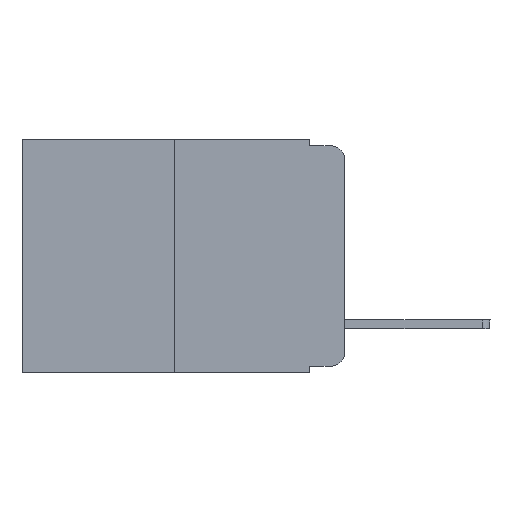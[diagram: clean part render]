
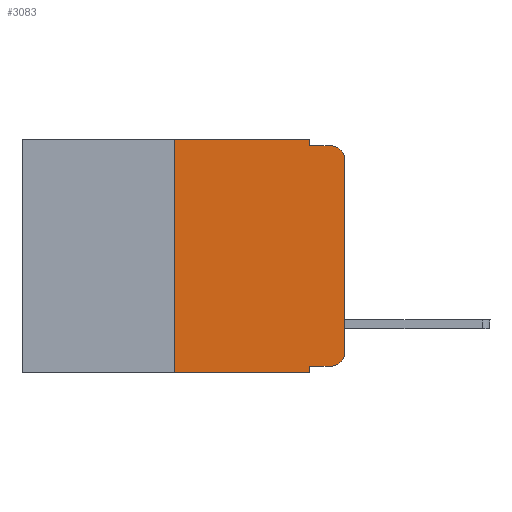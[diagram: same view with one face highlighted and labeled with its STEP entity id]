
A CAD part, left-side view. The second image highlights one B-rep face of the part: STEP entity #3083.
In plain terms, the highlighted planar face has unit normal (-1, 0, 0).
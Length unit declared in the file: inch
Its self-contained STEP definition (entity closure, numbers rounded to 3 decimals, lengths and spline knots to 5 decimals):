
#140 = DIRECTION ( 'NONE',  ( 0., -1., 0. ) ) ;
#408 = VERTEX_POINT ( 'NONE', #910 ) ;
#553 = ORIENTED_EDGE ( 'NONE', *, *, #4506, .T. ) ;
#562 = LINE ( 'NONE', #4885, #9786 ) ;
#564 = DIRECTION ( 'NONE',  ( 1., 0., 0. ) ) ;
#711 = EDGE_LOOP ( 'NONE', ( #5844, #2685, #13274, #2821, #1053, #6783, #12156, #6598, #553, #3997 ) ) ;
#843 = VERTEX_POINT ( 'NONE', #11855 ) ;
#910 = CARTESIAN_POINT ( 'NONE',  ( 0., 0.051, -0.01 ) ) ;
#1053 = ORIENTED_EDGE ( 'NONE', *, *, #3729, .F. ) ;
#1179 = VECTOR ( 'NONE', #4128, 39.37008 ) ;
#1207 = DIRECTION ( 'NONE',  ( 0., 0., -1. ) ) ;
#1239 = CARTESIAN_POINT ( 'NONE',  ( 0., 0.051, -0.333 ) ) ;
#1391 = CARTESIAN_POINT ( 'NONE',  ( 0., 0.25, 0. ) ) ;
#1409 = DIRECTION ( 'NONE',  ( 0., -1., 0. ) ) ;
#1519 = EDGE_CURVE ( 'NONE', #1644, #10442, #2931, .T. ) ;
#1644 = VERTEX_POINT ( 'NONE', #6235 ) ;
#1645 = DIRECTION ( 'NONE',  ( 0., -1., 0. ) ) ;
#1704 = VERTEX_POINT ( 'NONE', #1391 ) ;
#1884 = EDGE_CURVE ( 'NONE', #9315, #13483, #562, .T. ) ;
#2300 = LINE ( 'NONE', #12672, #10249 ) ;
#2417 = LINE ( 'NONE', #4503, #10703 ) ;
#2685 = ORIENTED_EDGE ( 'NONE', *, *, #12459, .T. ) ;
#2821 = ORIENTED_EDGE ( 'NONE', *, *, #6728, .F. ) ;
#2931 = CIRCLE ( 'NONE', #3819, 0.02 ) ;
#3071 = LINE ( 'NONE', #3214, #1179 ) ;
#3083 = ADVANCED_FACE ( 'NONE', ( #5799 ), #9998, .F. ) ;
#3214 = CARTESIAN_POINT ( 'NONE',  ( 0., 0.051, -0.01 ) ) ;
#3233 = CARTESIAN_POINT ( 'NONE',  ( 0., 0., -0.313 ) ) ;
#3527 = CARTESIAN_POINT ( 'NONE',  ( 0., 0.473, 0. ) ) ;
#3534 = LINE ( 'NONE', #6016, #8537 ) ;
#3564 = CARTESIAN_POINT ( 'NONE',  ( 0., 0.25, -0.343 ) ) ;
#3729 = EDGE_CURVE ( 'NONE', #1704, #4310, #6667, .T. ) ;
#3819 = AXIS2_PLACEMENT_3D ( 'NONE', #13474, #7956, #11334 ) ;
#3989 = EDGE_CURVE ( 'NONE', #8531, #13483, #2417, .T. ) ;
#3997 = ORIENTED_EDGE ( 'NONE', *, *, #1519, .T. ) ;
#4117 = AXIS2_PLACEMENT_3D ( 'NONE', #3527, #564, #7755 ) ;
#4128 = DIRECTION ( 'NONE',  ( 0., -1., 0. ) ) ;
#4310 = VERTEX_POINT ( 'NONE', #9295 ) ;
#4397 = CARTESIAN_POINT ( 'NONE',  ( 0., 0., 0. ) ) ;
#4503 = CARTESIAN_POINT ( 'NONE',  ( 0., 0.051, 0. ) ) ;
#4506 = EDGE_CURVE ( 'NONE', #8531, #1644, #8610, .T. ) ;
#4526 = LINE ( 'NONE', #4397, #7876 ) ;
#4885 = CARTESIAN_POINT ( 'NONE',  ( 0., 0.473, -0.343 ) ) ;
#5041 = EDGE_CURVE ( 'NONE', #10442, #843, #4526, .T. ) ;
#5357 = AXIS2_PLACEMENT_3D ( 'NONE', #6748, #9895, #1207 ) ;
#5652 = VECTOR ( 'NONE', #140, 39.37008 ) ;
#5691 = CARTESIAN_POINT ( 'NONE',  ( 0., 0.02, -0.01 ) ) ;
#5799 = FACE_OUTER_BOUND ( 'NONE', #711, .T. ) ;
#5844 = ORIENTED_EDGE ( 'NONE', *, *, #5041, .T. ) ;
#5941 = DIRECTION ( 'NONE',  ( 0., 0., 1. ) ) ;
#6016 = CARTESIAN_POINT ( 'NONE',  ( 0., 0.25, 0. ) ) ;
#6032 = CIRCLE ( 'NONE', #5357, 0.02 ) ;
#6235 = CARTESIAN_POINT ( 'NONE',  ( 0., 0.02, -0.333 ) ) ;
#6598 = ORIENTED_EDGE ( 'NONE', *, *, #3989, .F. ) ;
#6667 = LINE ( 'NONE', #10851, #11842 ) ;
#6728 = EDGE_CURVE ( 'NONE', #4310, #408, #2300, .T. ) ;
#6748 = CARTESIAN_POINT ( 'NONE',  ( 0., 0.02, -0.03 ) ) ;
#6783 = ORIENTED_EDGE ( 'NONE', *, *, #8504, .F. ) ;
#7566 = DIRECTION ( 'NONE',  ( 0., 0., 1. ) ) ;
#7683 = DIRECTION ( 'NONE',  ( 0., 0., -1. ) ) ;
#7755 = DIRECTION ( 'NONE',  ( 0., 0., -1. ) ) ;
#7876 = VECTOR ( 'NONE', #7566, 39.37008 ) ;
#7956 = DIRECTION ( 'NONE',  ( -1., 0., 0. ) ) ;
#8007 = CARTESIAN_POINT ( 'NONE',  ( 0., 0.051, -0.333 ) ) ;
#8504 = EDGE_CURVE ( 'NONE', #9315, #1704, #3534, .T. ) ;
#8531 = VERTEX_POINT ( 'NONE', #8007 ) ;
#8537 = VECTOR ( 'NONE', #5941, 39.37008 ) ;
#8610 = LINE ( 'NONE', #1239, #5652 ) ;
#9295 = CARTESIAN_POINT ( 'NONE',  ( 0., 0.051, 0. ) ) ;
#9315 = VERTEX_POINT ( 'NONE', #3564 ) ;
#9786 = VECTOR ( 'NONE', #1645, 39.37008 ) ;
#9895 = DIRECTION ( 'NONE',  ( -1., 0., 0. ) ) ;
#9998 = PLANE ( 'NONE',  #4117 ) ;
#10249 = VECTOR ( 'NONE', #10732, 39.37008 ) ;
#10442 = VERTEX_POINT ( 'NONE', #3233 ) ;
#10703 = VECTOR ( 'NONE', #7683, 39.37008 ) ;
#10732 = DIRECTION ( 'NONE',  ( 0., 0., -1. ) ) ;
#10851 = CARTESIAN_POINT ( 'NONE',  ( 0., 0.473, 0. ) ) ;
#10898 = EDGE_CURVE ( 'NONE', #408, #12514, #3071, .T. ) ;
#11334 = DIRECTION ( 'NONE',  ( 0., 0., -1. ) ) ;
#11842 = VECTOR ( 'NONE', #1409, 39.37008 ) ;
#11855 = CARTESIAN_POINT ( 'NONE',  ( 0., 0., -0.03 ) ) ;
#12156 = ORIENTED_EDGE ( 'NONE', *, *, #1884, .T. ) ;
#12459 = EDGE_CURVE ( 'NONE', #843, #12514, #6032, .T. ) ;
#12514 = VERTEX_POINT ( 'NONE', #5691 ) ;
#12672 = CARTESIAN_POINT ( 'NONE',  ( 0., 0.051, 0. ) ) ;
#13274 = ORIENTED_EDGE ( 'NONE', *, *, #10898, .F. ) ;
#13435 = CARTESIAN_POINT ( 'NONE',  ( 0., 0.051, -0.343 ) ) ;
#13474 = CARTESIAN_POINT ( 'NONE',  ( 0., 0.02, -0.313 ) ) ;
#13483 = VERTEX_POINT ( 'NONE', #13435 ) ;
